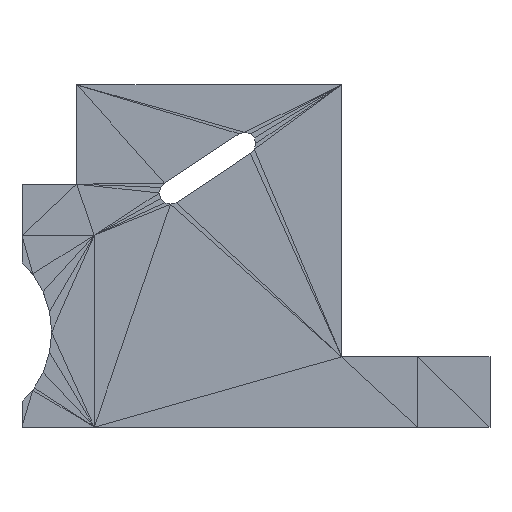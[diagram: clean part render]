
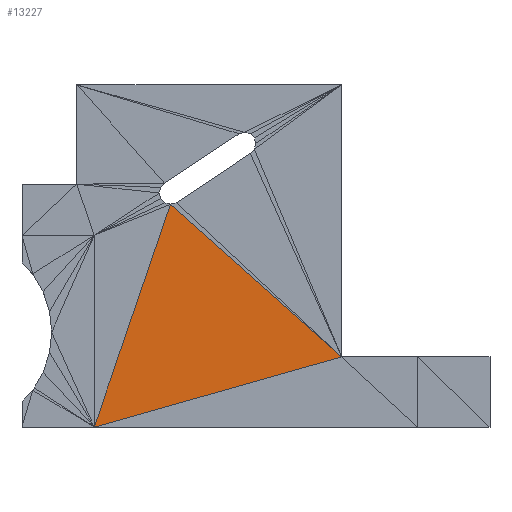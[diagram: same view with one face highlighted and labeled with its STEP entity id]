
A CAD part, top view. The second image highlights one B-rep face of the part: STEP entity #13227.
In plain terms, the highlighted planar face has unit normal (0, 0, 1).
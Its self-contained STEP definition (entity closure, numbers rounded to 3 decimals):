
#56 = VERTEX_POINT('',#57);
#57 = CARTESIAN_POINT('',(-9.525,6.89,3.047)
  );
#793 = VERTEX_POINT('',#794);
#794 = CARTESIAN_POINT('',(-19.304,-21.717,
    3.047));
#867 = PLANE('',#868);
#868 = AXIS2_PLACEMENT_3D('',#869,#870,#871);
#869 = CARTESIAN_POINT('',(2.027,-19.34,3.047)
  );
#870 = DIRECTION('',(0.,0.,1.));
#871 = DIRECTION('',(0.,1.,0.));
#11841 = VERTEX_POINT('',#11842);
#11842 = CARTESIAN_POINT('',(12.446,-12.7,
    3.047));
#12655 = PLANE('',#12656);
#12656 = AXIS2_PLACEMENT_3D('',#12657,#12658,#12659);
#12657 = CARTESIAN_POINT('',(1.503,-2.733,
    3.047));
#12658 = DIRECTION('',(0.,0.,1.));
#12659 = DIRECTION('',(0.,1.,0.));
#13201 = EDGE_CURVE('',#56,#11841,#13202,.T.);
#13202 = SURFACE_CURVE('',#13203,(#13207,#13214),.PCURVE_S1.);
#13203 = LINE('',#13204,#13205);
#13204 = CARTESIAN_POINT('',(-9.525,6.89,
    3.047));
#13205 = VECTOR('',#13206,1.);
#13206 = DIRECTION('',(0.746,-0.666,0.));
#13207 = PCURVE('',#12655,#13208);
#13208 = DEFINITIONAL_REPRESENTATION('',(#13209),#13213);
#13209 = LINE('',#13210,#13211);
#13210 = CARTESIAN_POINT('',(9.622,11.028));
#13211 = VECTOR('',#13212,1.);
#13212 = DIRECTION('',(-0.666,-0.746));
#13213 = ( GEOMETRIC_REPRESENTATION_CONTEXT(2) 
PARAMETRIC_REPRESENTATION_CONTEXT() REPRESENTATION_CONTEXT('2D SPACE',''
  ) );
#13214 = PCURVE('',#13215,#13220);
#13215 = PLANE('',#13216);
#13216 = AXIS2_PLACEMENT_3D('',#13217,#13218,#13219);
#13217 = CARTESIAN_POINT('',(-5.46,-9.47,
    3.047));
#13218 = DIRECTION('',(0.,0.,1.));
#13219 = DIRECTION('',(1.,0.,0.));
#13220 = DEFINITIONAL_REPRESENTATION('',(#13221),#13224);
#13221 = B_SPLINE_CURVE_WITH_KNOTS('',1,(#13222,#13223),.UNSPECIFIED.,
  .F.,.F.,(2,2),(0.,29.436),.PIECEWISE_BEZIER_KNOTS.);
#13222 = CARTESIAN_POINT('',(-4.065,16.36));
#13223 = CARTESIAN_POINT('',(17.906,-3.23));
#13224 = ( GEOMETRIC_REPRESENTATION_CONTEXT(2) 
PARAMETRIC_REPRESENTATION_CONTEXT() REPRESENTATION_CONTEXT('2D SPACE',''
  ) );
#13227 = ADVANCED_FACE('',(#13228),#13215,.T.);
#13228 = FACE_BOUND('',#13229,.T.);
#13229 = EDGE_LOOP('',(#13230,#13250,#13251));
#13230 = ORIENTED_EDGE('',*,*,#13231,.T.);
#13231 = EDGE_CURVE('',#793,#11841,#13232,.T.);
#13232 = SURFACE_CURVE('',#13233,(#13237,#13244),.PCURVE_S1.);
#13233 = LINE('',#13234,#13235);
#13234 = CARTESIAN_POINT('',(-19.304,-21.717,
    3.047));
#13235 = VECTOR('',#13236,1.);
#13236 = DIRECTION('',(0.962,0.273,0.));
#13237 = PCURVE('',#13215,#13238);
#13238 = DEFINITIONAL_REPRESENTATION('',(#13239),#13243);
#13239 = LINE('',#13240,#13241);
#13240 = CARTESIAN_POINT('',(-13.844,-12.247));
#13241 = VECTOR('',#13242,1.);
#13242 = DIRECTION('',(0.962,0.273));
#13243 = ( GEOMETRIC_REPRESENTATION_CONTEXT(2) 
PARAMETRIC_REPRESENTATION_CONTEXT() REPRESENTATION_CONTEXT('2D SPACE',''
  ) );
#13244 = PCURVE('',#867,#13245);
#13245 = DEFINITIONAL_REPRESENTATION('',(#13246),#13249);
#13246 = B_SPLINE_CURVE_WITH_KNOTS('',1,(#13247,#13248),.UNSPECIFIED.,
  .F.,.F.,(2,2),(0.,33.005),.PIECEWISE_BEZIER_KNOTS.);
#13247 = CARTESIAN_POINT('',(-2.377,21.331));
#13248 = CARTESIAN_POINT('',(6.64,-10.419));
#13249 = ( GEOMETRIC_REPRESENTATION_CONTEXT(2) 
PARAMETRIC_REPRESENTATION_CONTEXT() REPRESENTATION_CONTEXT('2D SPACE',''
  ) );
#13250 = ORIENTED_EDGE('',*,*,#13201,.F.);
#13251 = ORIENTED_EDGE('',*,*,#13252,.T.);
#13252 = EDGE_CURVE('',#56,#793,#13253,.T.);
#13253 = SURFACE_CURVE('',#13254,(#13258,#13265),.PCURVE_S1.);
#13254 = LINE('',#13255,#13256);
#13255 = CARTESIAN_POINT('',(-9.525,6.89,
    3.047));
#13256 = VECTOR('',#13257,1.);
#13257 = DIRECTION('',(-0.323,-0.946,0.));
#13258 = PCURVE('',#13215,#13259);
#13259 = DEFINITIONAL_REPRESENTATION('',(#13260),#13264);
#13260 = LINE('',#13261,#13262);
#13261 = CARTESIAN_POINT('',(-4.065,16.36));
#13262 = VECTOR('',#13263,1.);
#13263 = DIRECTION('',(-0.323,-0.946));
#13264 = ( GEOMETRIC_REPRESENTATION_CONTEXT(2) 
PARAMETRIC_REPRESENTATION_CONTEXT() REPRESENTATION_CONTEXT('2D SPACE',''
  ) );
#13265 = PCURVE('',#13266,#13271);
#13266 = PLANE('',#13267);
#13267 = AXIS2_PLACEMENT_3D('',#13268,#13269,#13270);
#13268 = CARTESIAN_POINT('',(-16.256,-6.174,
    3.047));
#13269 = DIRECTION('',(0.,0.,1.));
#13270 = DIRECTION('',(1.,0.,0.));
#13271 = DEFINITIONAL_REPRESENTATION('',(#13272),#13275);
#13272 = B_SPLINE_CURVE_WITH_KNOTS('',1,(#13273,#13274),.UNSPECIFIED.,
  .F.,.F.,(2,2),(0.,30.232),.PIECEWISE_BEZIER_KNOTS.);
#13273 = CARTESIAN_POINT('',(6.731,13.064));
#13274 = CARTESIAN_POINT('',(-3.048,-15.543));
#13275 = ( GEOMETRIC_REPRESENTATION_CONTEXT(2) 
PARAMETRIC_REPRESENTATION_CONTEXT() REPRESENTATION_CONTEXT('2D SPACE',''
  ) );
